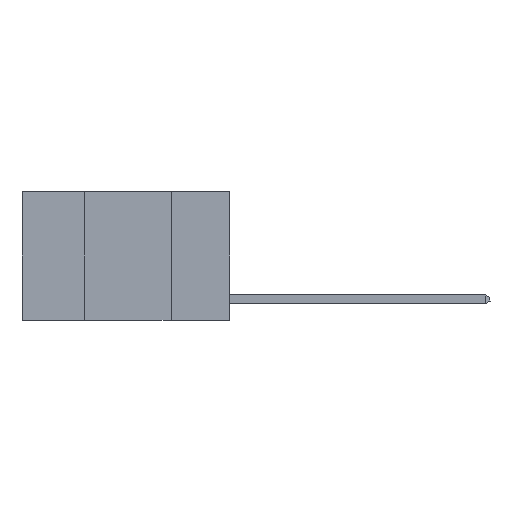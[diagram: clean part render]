
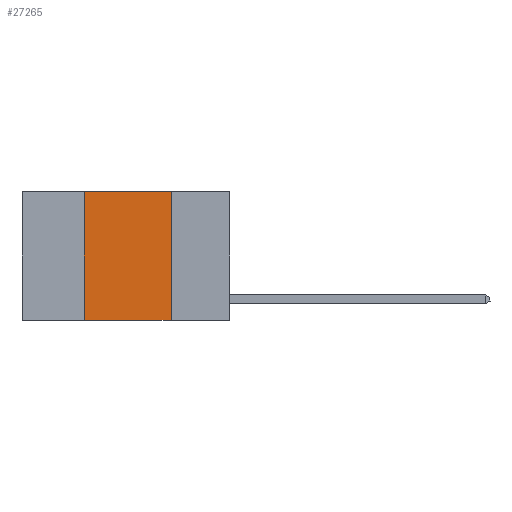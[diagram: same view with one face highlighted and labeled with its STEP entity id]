
A CAD part, left-side view. The second image highlights one B-rep face of the part: STEP entity #27265.
In plain terms, the highlighted planar face has unit normal (-1, 0, 0).
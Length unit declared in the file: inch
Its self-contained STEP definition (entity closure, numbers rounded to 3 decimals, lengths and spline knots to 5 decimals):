
#304 = PLANE ( 'NONE',  #27530 ) ;
#372 = VECTOR ( 'NONE', #14568, 39.37008 ) ;
#1370 = CARTESIAN_POINT ( 'NONE',  ( 0., 0.42, -0.37 ) ) ;
#1621 = CARTESIAN_POINT ( 'NONE',  ( 0., 0.6, -0.37 ) ) ;
#2250 = EDGE_CURVE ( 'NONE', #5553, #5768, #5237, .T. ) ;
#3079 = CARTESIAN_POINT ( 'NONE',  ( 0., 0.17, 0. ) ) ;
#4810 = EDGE_CURVE ( 'NONE', #19505, #5768, #21334, .T. ) ;
#5237 = LINE ( 'NONE', #1621, #11588 ) ;
#5553 = VERTEX_POINT ( 'NONE', #1370 ) ;
#5768 = VERTEX_POINT ( 'NONE', #8027 ) ;
#5809 = DIRECTION ( 'NONE',  ( 0., 0., -1. ) ) ;
#6717 = DIRECTION ( 'NONE',  ( 1., 0., 0. ) ) ;
#7620 = ORIENTED_EDGE ( 'NONE', *, *, #2250, .T. ) ;
#7899 = DIRECTION ( 'NONE',  ( 0., -1., 0. ) ) ;
#8027 = CARTESIAN_POINT ( 'NONE',  ( 0., 0.17, -0.37 ) ) ;
#8114 = LINE ( 'NONE', #16521, #372 ) ;
#8518 = VECTOR ( 'NONE', #5809, 39.37008 ) ;
#8725 = ORIENTED_EDGE ( 'NONE', *, *, #26318, .F. ) ;
#8782 = DIRECTION ( 'NONE',  ( 0., 0., -1. ) ) ;
#10479 = CARTESIAN_POINT ( 'NONE',  ( 0., 0.17, 0. ) ) ;
#11588 = VECTOR ( 'NONE', #7899, 39.37008 ) ;
#11631 = VECTOR ( 'NONE', #25519, 39.37008 ) ;
#12674 = LINE ( 'NONE', #21209, #11631 ) ;
#12743 = VERTEX_POINT ( 'NONE', #27396 ) ;
#13029 = ORIENTED_EDGE ( 'NONE', *, *, #4810, .F. ) ;
#14338 = ORIENTED_EDGE ( 'NONE', *, *, #20631, .F. ) ;
#14568 = DIRECTION ( 'NONE',  ( 0., 0., 1. ) ) ;
#16521 = CARTESIAN_POINT ( 'NONE',  ( 0., 0.42, 0. ) ) ;
#19505 = VERTEX_POINT ( 'NONE', #3079 ) ;
#20631 = EDGE_CURVE ( 'NONE', #12743, #19505, #12674, .T. ) ;
#21209 = CARTESIAN_POINT ( 'NONE',  ( 0., 0.6, 0. ) ) ;
#21334 = LINE ( 'NONE', #10479, #8518 ) ;
#21620 = EDGE_LOOP ( 'NONE', ( #13029, #14338, #8725, #7620 ) ) ;
#21672 = CARTESIAN_POINT ( 'NONE',  ( 0., 0.6, 0. ) ) ;
#25519 = DIRECTION ( 'NONE',  ( 0., -1., 0. ) ) ;
#25696 = FACE_OUTER_BOUND ( 'NONE', #21620, .T. ) ;
#26318 = EDGE_CURVE ( 'NONE', #5553, #12743, #8114, .T. ) ;
#27265 = ADVANCED_FACE ( 'NONE', ( #25696 ), #304, .F. ) ;
#27396 = CARTESIAN_POINT ( 'NONE',  ( 0., 0.42, 0. ) ) ;
#27530 = AXIS2_PLACEMENT_3D ( 'NONE', #21672, #6717, #8782 ) ;
